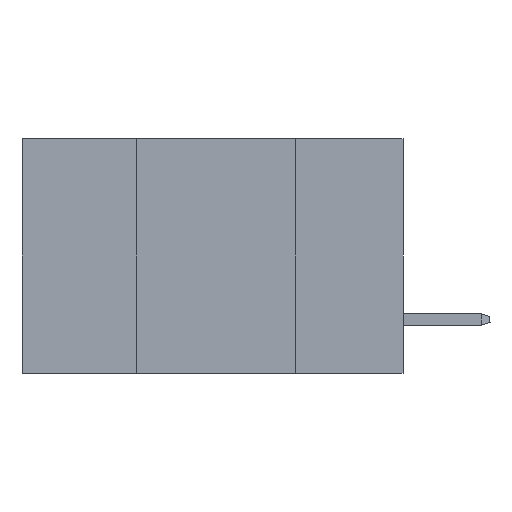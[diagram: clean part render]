
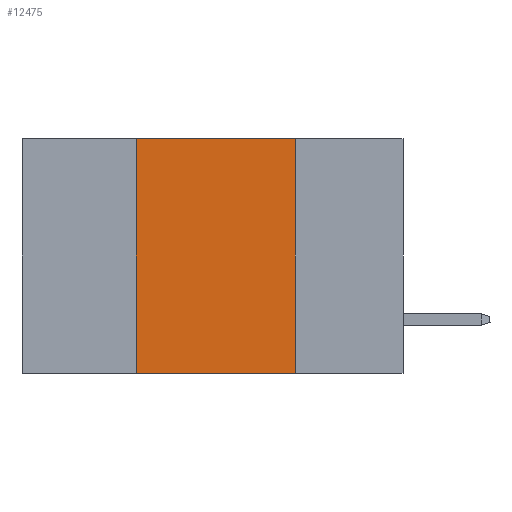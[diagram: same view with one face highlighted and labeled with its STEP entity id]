
A CAD part, left-side view. The second image highlights one B-rep face of the part: STEP entity #12475.
In plain terms, the highlighted planar face has unit normal (-1, 0, 0).
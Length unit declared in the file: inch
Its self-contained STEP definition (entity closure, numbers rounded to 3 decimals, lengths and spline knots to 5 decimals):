
#2385 = CARTESIAN_POINT ( 'NONE',  ( 0., 0.6, 0. ) ) ;
#4493 = CARTESIAN_POINT ( 'NONE',  ( 0., 0.6, 0. ) ) ;
#4817 = EDGE_CURVE ( 'NONE', #16445, #26464, #44117, .T. ) ;
#10321 = VECTOR ( 'NONE', #16199, 39.37008 ) ;
#10945 = ORIENTED_EDGE ( 'NONE', *, *, #4817, .F. ) ;
#11959 = CARTESIAN_POINT ( 'NONE',  ( 0., 0.42, -0.37 ) ) ;
#12475 = ADVANCED_FACE ( 'NONE', ( #28523 ), #18533, .F. ) ;
#14334 = EDGE_CURVE ( 'NONE', #35448, #16445, #22787, .T. ) ;
#16106 = VERTEX_POINT ( 'NONE', #11959 ) ;
#16132 = DIRECTION ( 'NONE',  ( 0., 0., 1. ) ) ;
#16199 = DIRECTION ( 'NONE',  ( 0., -1., 0. ) ) ;
#16354 = LINE ( 'NONE', #19981, #16706 ) ;
#16445 = VERTEX_POINT ( 'NONE', #37774 ) ;
#16706 = VECTOR ( 'NONE', #36762, 39.37008 ) ;
#17861 = DIRECTION ( 'NONE',  ( 1., 0., 0. ) ) ;
#18533 = PLANE ( 'NONE',  #43521 ) ;
#19981 = CARTESIAN_POINT ( 'NONE',  ( 0., 0.6, -0.37 ) ) ;
#22787 = LINE ( 'NONE', #2385, #10321 ) ;
#22812 = ORIENTED_EDGE ( 'NONE', *, *, #25183, .T. ) ;
#22950 = CARTESIAN_POINT ( 'NONE',  ( 0., 0.42, 0. ) ) ;
#25183 = EDGE_CURVE ( 'NONE', #16106, #26464, #16354, .T. ) ;
#26464 = VERTEX_POINT ( 'NONE', #36317 ) ;
#26880 = CARTESIAN_POINT ( 'NONE',  ( 0., 0.17, 0. ) ) ;
#28523 = FACE_OUTER_BOUND ( 'NONE', #31264, .T. ) ;
#28966 = DIRECTION ( 'NONE',  ( 0., 0., -1. ) ) ;
#31264 = EDGE_LOOP ( 'NONE', ( #10945, #41468, #43143, #22812 ) ) ;
#32930 = LINE ( 'NONE', #22950, #41743 ) ;
#34928 = EDGE_CURVE ( 'NONE', #16106, #35448, #32930, .T. ) ;
#35448 = VERTEX_POINT ( 'NONE', #39816 ) ;
#36183 = DIRECTION ( 'NONE',  ( 0., 0., -1. ) ) ;
#36317 = CARTESIAN_POINT ( 'NONE',  ( 0., 0.17, -0.37 ) ) ;
#36762 = DIRECTION ( 'NONE',  ( 0., -1., 0. ) ) ;
#37774 = CARTESIAN_POINT ( 'NONE',  ( 0., 0.17, 0. ) ) ;
#39816 = CARTESIAN_POINT ( 'NONE',  ( 0., 0.42, 0. ) ) ;
#41468 = ORIENTED_EDGE ( 'NONE', *, *, #14334, .F. ) ;
#41743 = VECTOR ( 'NONE', #16132, 39.37008 ) ;
#43143 = ORIENTED_EDGE ( 'NONE', *, *, #34928, .F. ) ;
#43521 = AXIS2_PLACEMENT_3D ( 'NONE', #4493, #17861, #28966 ) ;
#43942 = VECTOR ( 'NONE', #36183, 39.37008 ) ;
#44117 = LINE ( 'NONE', #26880, #43942 ) ;
